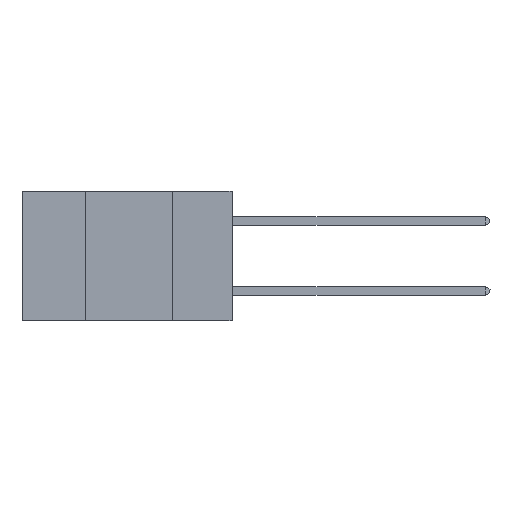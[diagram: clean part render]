
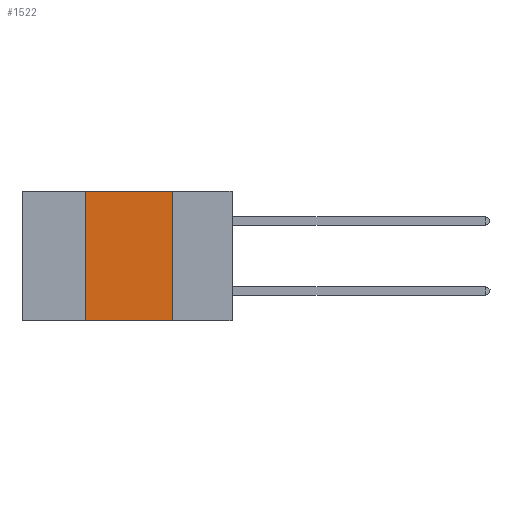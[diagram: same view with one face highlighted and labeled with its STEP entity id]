
A CAD part, left-side view. The second image highlights one B-rep face of the part: STEP entity #1522.
In plain terms, the highlighted planar face has unit normal (-1, 0, 0).
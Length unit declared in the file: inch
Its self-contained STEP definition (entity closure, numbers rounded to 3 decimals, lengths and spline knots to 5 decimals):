
#12 = VERTEX_POINT ( 'NONE', #7207 ) ;
#85 = EDGE_CURVE ( 'NONE', #8146, #4960, #1850, .T. ) ;
#927 = ORIENTED_EDGE ( 'NONE', *, *, #6547, .F. ) ;
#1075 = ORIENTED_EDGE ( 'NONE', *, *, #85, .F. ) ;
#1469 = AXIS2_PLACEMENT_3D ( 'NONE', #6201, #10254, #7749 ) ;
#1522 = ADVANCED_FACE ( 'NONE', ( #8614 ), #8703, .F. ) ;
#1850 = LINE ( 'NONE', #8776, #5923 ) ;
#2796 = CARTESIAN_POINT ( 'NONE',  ( 0., 0.17, -0.37 ) ) ;
#2802 = DIRECTION ( 'NONE',  ( 0., -1., 0. ) ) ;
#2986 = VECTOR ( 'NONE', #6099, 39.37008 ) ;
#3079 = DIRECTION ( 'NONE',  ( 0., -1., 0. ) ) ;
#3119 = ORIENTED_EDGE ( 'NONE', *, *, #5466, .T. ) ;
#3557 = CARTESIAN_POINT ( 'NONE',  ( 0., 0.6, 0. ) ) ;
#3646 = VECTOR ( 'NONE', #3079, 39.37008 ) ;
#3665 = ORIENTED_EDGE ( 'NONE', *, *, #8456, .F. ) ;
#3948 = CARTESIAN_POINT ( 'NONE',  ( 0., 0.42, -0.37 ) ) ;
#4099 = LINE ( 'NONE', #4568, #2986 ) ;
#4133 = VECTOR ( 'NONE', #2802, 39.37008 ) ;
#4568 = CARTESIAN_POINT ( 'NONE',  ( 0., 0.17, 0. ) ) ;
#4960 = VERTEX_POINT ( 'NONE', #6140 ) ;
#4992 = LINE ( 'NONE', #7863, #3646 ) ;
#5466 = EDGE_CURVE ( 'NONE', #8146, #8359, #4992, .T. ) ;
#5923 = VECTOR ( 'NONE', #9589, 39.37008 ) ;
#6099 = DIRECTION ( 'NONE',  ( 0., 0., -1. ) ) ;
#6140 = CARTESIAN_POINT ( 'NONE',  ( 0., 0.42, 0. ) ) ;
#6201 = CARTESIAN_POINT ( 'NONE',  ( 0., 0.6, 0. ) ) ;
#6547 = EDGE_CURVE ( 'NONE', #4960, #12, #7219, .T. ) ;
#7207 = CARTESIAN_POINT ( 'NONE',  ( 0., 0.17, 0. ) ) ;
#7219 = LINE ( 'NONE', #3557, #4133 ) ;
#7749 = DIRECTION ( 'NONE',  ( 0., 0., -1. ) ) ;
#7863 = CARTESIAN_POINT ( 'NONE',  ( 0., 0.6, -0.37 ) ) ;
#8071 = EDGE_LOOP ( 'NONE', ( #3665, #927, #1075, #3119 ) ) ;
#8146 = VERTEX_POINT ( 'NONE', #3948 ) ;
#8359 = VERTEX_POINT ( 'NONE', #2796 ) ;
#8456 = EDGE_CURVE ( 'NONE', #12, #8359, #4099, .T. ) ;
#8614 = FACE_OUTER_BOUND ( 'NONE', #8071, .T. ) ;
#8703 = PLANE ( 'NONE',  #1469 ) ;
#8776 = CARTESIAN_POINT ( 'NONE',  ( 0., 0.42, 0. ) ) ;
#9589 = DIRECTION ( 'NONE',  ( 0., 0., 1. ) ) ;
#10254 = DIRECTION ( 'NONE',  ( 1., 0., 0. ) ) ;
